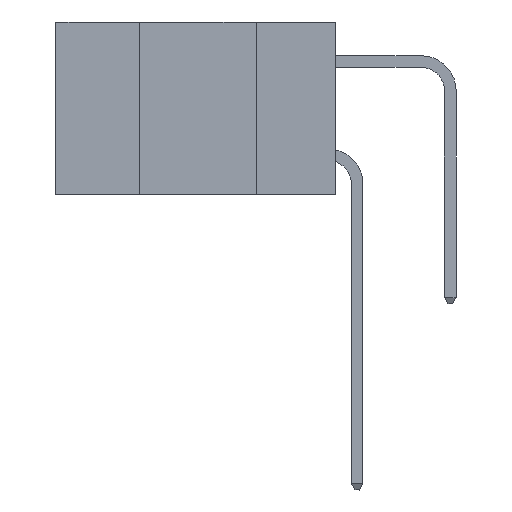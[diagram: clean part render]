
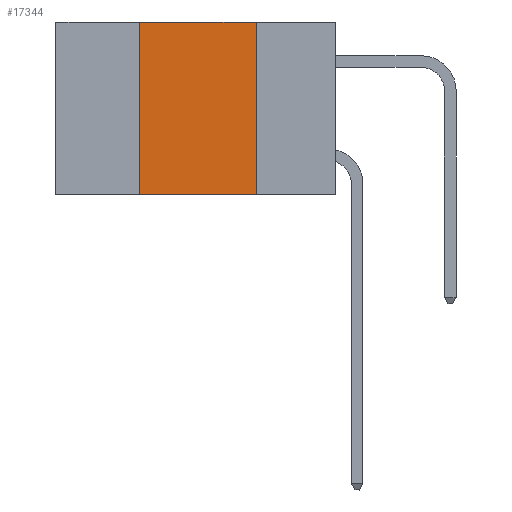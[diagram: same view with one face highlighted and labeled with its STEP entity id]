
A CAD part, left-side view. The second image highlights one B-rep face of the part: STEP entity #17344.
In plain terms, the highlighted planar face has unit normal (-1, 0, 0).
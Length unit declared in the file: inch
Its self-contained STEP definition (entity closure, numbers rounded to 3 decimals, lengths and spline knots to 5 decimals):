
#414 = AXIS2_PLACEMENT_3D ( 'NONE', #14690, #8427, #5138 ) ;
#867 = VERTEX_POINT ( 'NONE', #6253 ) ;
#1054 = EDGE_CURVE ( 'NONE', #20570, #12259, #13460, .T. ) ;
#1329 = VERTEX_POINT ( 'NONE', #11219 ) ;
#1858 = FACE_OUTER_BOUND ( 'NONE', #20687, .T. ) ;
#2022 = ORIENTED_EDGE ( 'NONE', *, *, #17130, .F. ) ;
#3374 = ORIENTED_EDGE ( 'NONE', *, *, #1054, .T. ) ;
#3474 = DIRECTION ( 'NONE',  ( 0., 0., 1. ) ) ;
#4801 = ORIENTED_EDGE ( 'NONE', *, *, #8850, .F. ) ;
#5138 = DIRECTION ( 'NONE',  ( 0., 0., -1. ) ) ;
#5679 = VECTOR ( 'NONE', #3474, 39.37008 ) ;
#6253 = CARTESIAN_POINT ( 'NONE',  ( 0., 0.42, 0. ) ) ;
#6943 = PLANE ( 'NONE',  #414 ) ;
#7197 = DIRECTION ( 'NONE',  ( 0., -1., 0. ) ) ;
#8427 = DIRECTION ( 'NONE',  ( 1., 0., 0. ) ) ;
#8850 = EDGE_CURVE ( 'NONE', #20570, #867, #17953, .T. ) ;
#9487 = VECTOR ( 'NONE', #7197, 39.37008 ) ;
#10892 = CARTESIAN_POINT ( 'NONE',  ( 0., 0.17, 0. ) ) ;
#11219 = CARTESIAN_POINT ( 'NONE',  ( 0., 0.17, 0. ) ) ;
#11583 = CARTESIAN_POINT ( 'NONE',  ( 0., 0.17, -0.37 ) ) ;
#11927 = VECTOR ( 'NONE', #12072, 39.37008 ) ;
#12072 = DIRECTION ( 'NONE',  ( 0., 0., -1. ) ) ;
#12259 = VERTEX_POINT ( 'NONE', #11583 ) ;
#12394 = ORIENTED_EDGE ( 'NONE', *, *, #17205, .F. ) ;
#12804 = LINE ( 'NONE', #20798, #15948 ) ;
#13460 = LINE ( 'NONE', #19978, #9487 ) ;
#14690 = CARTESIAN_POINT ( 'NONE',  ( 0., 0.6, 0. ) ) ;
#14910 = CARTESIAN_POINT ( 'NONE',  ( 0., 0.42, 0. ) ) ;
#15948 = VECTOR ( 'NONE', #16156, 39.37008 ) ;
#16156 = DIRECTION ( 'NONE',  ( 0., -1., 0. ) ) ;
#17118 = LINE ( 'NONE', #10892, #11927 ) ;
#17130 = EDGE_CURVE ( 'NONE', #1329, #12259, #17118, .T. ) ;
#17205 = EDGE_CURVE ( 'NONE', #867, #1329, #12804, .T. ) ;
#17344 = ADVANCED_FACE ( 'NONE', ( #1858 ), #6943, .F. ) ;
#17953 = LINE ( 'NONE', #14910, #5679 ) ;
#19978 = CARTESIAN_POINT ( 'NONE',  ( 0., 0.6, -0.37 ) ) ;
#20157 = CARTESIAN_POINT ( 'NONE',  ( 0., 0.42, -0.37 ) ) ;
#20570 = VERTEX_POINT ( 'NONE', #20157 ) ;
#20687 = EDGE_LOOP ( 'NONE', ( #2022, #12394, #4801, #3374 ) ) ;
#20798 = CARTESIAN_POINT ( 'NONE',  ( 0., 0.6, 0. ) ) ;
